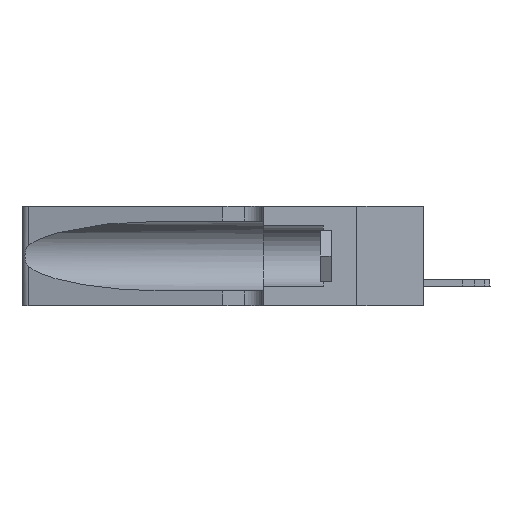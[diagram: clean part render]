
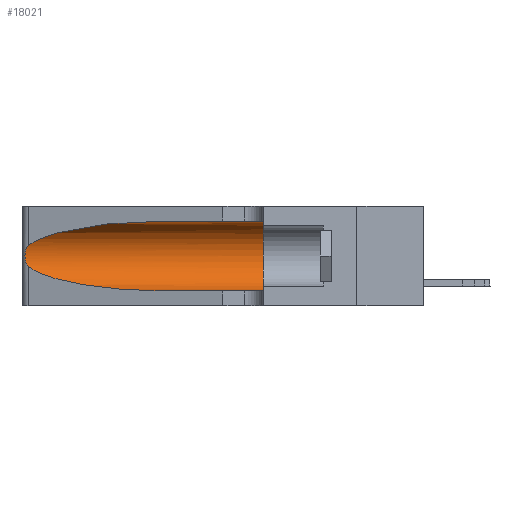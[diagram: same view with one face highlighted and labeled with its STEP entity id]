
A CAD part, left-side view. The second image highlights one B-rep face of the part: STEP entity #18021.
In plain terms, the highlighted cylindrical face has radius 3.308 mm (diameter 6.617 mm), a partial arc.
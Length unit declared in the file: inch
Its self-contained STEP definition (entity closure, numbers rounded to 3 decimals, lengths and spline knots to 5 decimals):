
#560 = DIRECTION ( 'NONE',  ( 0., 0., 1. ) ) ;
#617 = EDGE_LOOP ( 'NONE', ( #24545, #12226, #26085, #14510, #17003, #13535 ) ) ;
#623 = FACE_OUTER_BOUND ( 'NONE', #617, .T. ) ;
#1732 = EDGE_CURVE ( 'NONE', #5619, #19730, #17468, .T. ) ;
#1920 =( BOUNDED_CURVE ( )  B_SPLINE_CURVE ( 3, ( #5125, #9409, #11607, #24813 ),
 .UNSPECIFIED., .F., .F. ) 
 B_SPLINE_CURVE_WITH_KNOTS ( ( 4, 4 ),
 ( 3.44316, 4.71239 ),
 .UNSPECIFIED. ) 
 CURVE ( )  GEOMETRIC_REPRESENTATION_ITEM ( )  RATIONAL_B_SPLINE_CURVE ( ( 1., 0.87, 0.87, 1. ) ) 
 REPRESENTATION_ITEM ( '' )  );
#2023 = VERTEX_POINT ( 'NONE', #15974 ) ;
#2070 = CARTESIAN_POINT ( 'NONE',  ( 0.1305, 0.72297, 0.31525 ) ) ;
#2555 = AXIS2_PLACEMENT_3D ( 'NONE', #19231, #6199, #8577 ) ;
#2903 = CARTESIAN_POINT ( 'NONE',  ( 0.25854, 1.2359, 0.20912 ) ) ;
#3472 = AXIS2_PLACEMENT_3D ( 'NONE', #13600, #13891, #560 ) ;
#3847 = LINE ( 'NONE', #19906, #26650 ) ;
#5125 = CARTESIAN_POINT ( 'NONE',  ( 0.25487, 1.22718, 0.14631 ) ) ;
#5619 = VERTEX_POINT ( 'NONE', #22075 ) ;
#6071 = B_SPLINE_CURVE_WITH_KNOTS ( 'NONE', 3,
 ( #18784, #18875, #23330, #12606, #2903, #21186, #12250, #7181, #21092, #8054, #23358, #12722, #25574, #19169 ),
 .UNSPECIFIED., .F., .F.,
 ( 4, 2, 2, 2, 2, 2, 4 ),
 ( 0., 0.00027, 0.00053, 0.00107, 0.0016, 0.00187, 0.00214 ),
 .UNSPECIFIED. ) ;
#6199 = DIRECTION ( 'NONE',  ( 0., -1., 0. ) ) ;
#7181 = CARTESIAN_POINT ( 'NONE',  ( 0.26075, 1.23896, 0.178 ) ) ;
#7238 = CARTESIAN_POINT ( 'NONE',  ( 0.1305, 0.72297, 0.05475 ) ) ;
#7383 = CIRCLE ( 'NONE', #3472, 0.13025 ) ;
#7722 = CARTESIAN_POINT ( 'NONE',  ( 0.1305, 0.35, 0.05475 ) ) ;
#7912 = EDGE_CURVE ( 'NONE', #8371, #11712, #3847, .T. ) ;
#8054 = CARTESIAN_POINT ( 'NONE',  ( 0.25856, 1.23593, 0.16098 ) ) ;
#8371 = VERTEX_POINT ( 'NONE', #7238 ) ;
#8577 = DIRECTION ( 'NONE',  ( 0., 0., -1. ) ) ;
#9198 = CARTESIAN_POINT ( 'NONE',  ( 0.1305, 0.35, 0.31525 ) ) ;
#9409 = CARTESIAN_POINT ( 'NONE',  ( 0.2373, 1.15595, 0.08982 ) ) ;
#9942 = CARTESIAN_POINT ( 'NONE',  ( 0.25487, 1.22718, 0.22369 ) ) ;
#10355 = CARTESIAN_POINT ( 'NONE',  ( 0.1305, 1.61858, 0.31525 ) ) ;
#11607 = CARTESIAN_POINT ( 'NONE',  ( 0.18966, 0.96281, 0.05475 ) ) ;
#11712 = VERTEX_POINT ( 'NONE', #7722 ) ;
#12219 = CARTESIAN_POINT ( 'NONE',  ( 0.2373, 1.15595, 0.28018 ) ) ;
#12226 = ORIENTED_EDGE ( 'NONE', *, *, #15074, .T. ) ;
#12250 = CARTESIAN_POINT ( 'NONE',  ( 0.26075, 1.23896, 0.19203 ) ) ;
#12317 = CARTESIAN_POINT ( 'NONE',  ( 0.18966, 0.96281, 0.31525 ) ) ;
#12350 = DIRECTION ( 'NONE',  ( 0., -1., 0. ) ) ;
#12606 = CARTESIAN_POINT ( 'NONE',  ( 0.25787, 1.23484, 0.2124 ) ) ;
#12722 = CARTESIAN_POINT ( 'NONE',  ( 0.25639, 1.23186, 0.15144 ) ) ;
#13355 = DIRECTION ( 'NONE',  ( 0., -1., 0. ) ) ;
#13535 = ORIENTED_EDGE ( 'NONE', *, *, #1732, .F. ) ;
#13600 = CARTESIAN_POINT ( 'NONE',  ( 0.1305, 0.35, 0.185 ) ) ;
#13891 = DIRECTION ( 'NONE',  ( 0., 1., 0. ) ) ;
#14510 = ORIENTED_EDGE ( 'NONE', *, *, #7912, .T. ) ;
#15074 = EDGE_CURVE ( 'NONE', #2023, #15891, #6071, .T. ) ;
#15891 = VERTEX_POINT ( 'NONE', #16331 ) ;
#15974 = CARTESIAN_POINT ( 'NONE',  ( 0.25487, 1.22718, 0.22369 ) ) ;
#16331 = CARTESIAN_POINT ( 'NONE',  ( 0.25487, 1.22718, 0.14631 ) ) ;
#17003 = ORIENTED_EDGE ( 'NONE', *, *, #28130, .F. ) ;
#17468 = LINE ( 'NONE', #10355, #26997 ) ;
#18021 = ADVANCED_FACE ( 'NONE', ( #623 ), #20366, .F. ) ;
#18784 = CARTESIAN_POINT ( 'NONE',  ( 0.25487, 1.22718, 0.22369 ) ) ;
#18875 = CARTESIAN_POINT ( 'NONE',  ( 0.25555, 1.22994, 0.2215 ) ) ;
#19169 = CARTESIAN_POINT ( 'NONE',  ( 0.25487, 1.22718, 0.14631 ) ) ;
#19231 = CARTESIAN_POINT ( 'NONE',  ( 0.1305, 1.61858, 0.185 ) ) ;
#19730 = VERTEX_POINT ( 'NONE', #9198 ) ;
#19906 = CARTESIAN_POINT ( 'NONE',  ( 0.1305, 1.61858, 0.05475 ) ) ;
#20366 = CYLINDRICAL_SURFACE ( 'NONE', #2555, 0.13025 ) ;
#21092 = CARTESIAN_POINT ( 'NONE',  ( 0.26017, 1.23833, 0.17102 ) ) ;
#21186 = CARTESIAN_POINT ( 'NONE',  ( 0.26018, 1.23835, 0.19895 ) ) ;
#22075 = CARTESIAN_POINT ( 'NONE',  ( 0.1305, 0.72297, 0.31525 ) ) ;
#23119 = EDGE_CURVE ( 'NONE', #5619, #2023, #26668, .T. ) ;
#23330 = CARTESIAN_POINT ( 'NONE',  ( 0.25639, 1.23184, 0.21858 ) ) ;
#23358 = CARTESIAN_POINT ( 'NONE',  ( 0.25789, 1.23486, 0.15765 ) ) ;
#24545 = ORIENTED_EDGE ( 'NONE', *, *, #23119, .T. ) ;
#24813 = CARTESIAN_POINT ( 'NONE',  ( 0.1305, 0.72297, 0.05475 ) ) ;
#25574 = CARTESIAN_POINT ( 'NONE',  ( 0.25555, 1.22993, 0.14849 ) ) ;
#25803 = EDGE_CURVE ( 'NONE', #15891, #8371, #1920, .T. ) ;
#26085 = ORIENTED_EDGE ( 'NONE', *, *, #25803, .T. ) ;
#26650 = VECTOR ( 'NONE', #13355, 39.37008 ) ;
#26668 =( BOUNDED_CURVE ( )  B_SPLINE_CURVE ( 3, ( #2070, #12317, #12219, #9942 ),
 .UNSPECIFIED., .F., .T. ) 
 B_SPLINE_CURVE_WITH_KNOTS ( ( 4, 4 ),
 ( 1.5708, 2.84003 ),
 .UNSPECIFIED. ) 
 CURVE ( )  GEOMETRIC_REPRESENTATION_ITEM ( )  RATIONAL_B_SPLINE_CURVE ( ( 1., 0.87, 0.87, 1. ) ) 
 REPRESENTATION_ITEM ( '' )  );
#26997 = VECTOR ( 'NONE', #12350, 39.37008 ) ;
#28130 = EDGE_CURVE ( 'NONE', #19730, #11712, #7383, .T. ) ;
